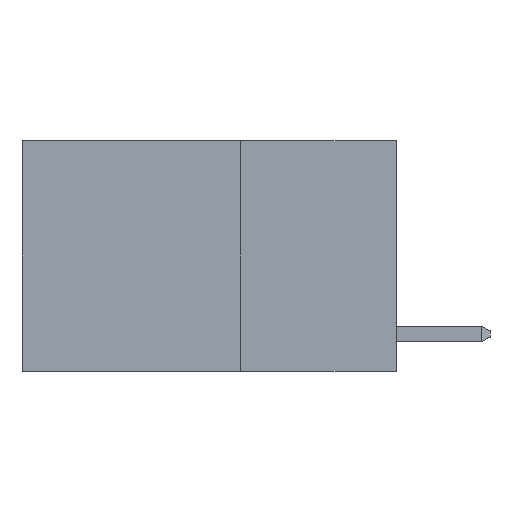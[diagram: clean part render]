
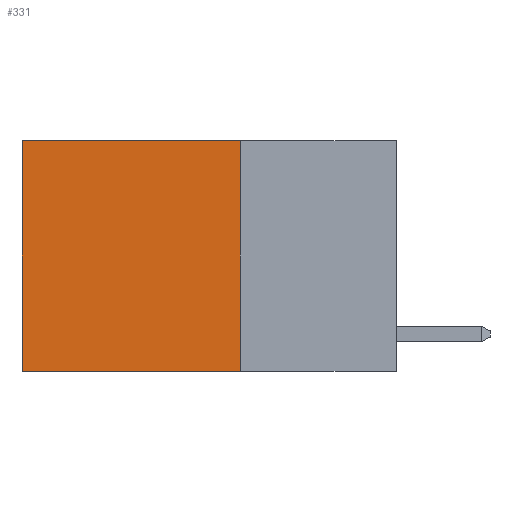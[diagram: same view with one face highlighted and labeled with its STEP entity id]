
A CAD part, left-side view. The second image highlights one B-rep face of the part: STEP entity #331.
In plain terms, the highlighted planar face has unit normal (-1, 0, 0).
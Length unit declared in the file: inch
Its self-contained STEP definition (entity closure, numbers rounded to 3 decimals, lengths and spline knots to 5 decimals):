
#331 = ADVANCED_FACE ( 'NONE', ( #4762 ), #3990, .F. ) ;
#354 = DIRECTION ( 'NONE',  ( 0., 0., -1. ) ) ;
#567 = CARTESIAN_POINT ( 'NONE',  ( 0.2625, 0.25, 0. ) ) ;
#941 = VERTEX_POINT ( 'NONE', #567 ) ;
#1017 = LINE ( 'NONE', #2188, #1271 ) ;
#1229 = EDGE_LOOP ( 'NONE', ( #3267, #4927, #3034, #3205 ) ) ;
#1271 = VECTOR ( 'NONE', #3035, 39.37008 ) ;
#1307 = VERTEX_POINT ( 'NONE', #6038 ) ;
#2188 = CARTESIAN_POINT ( 'NONE',  ( 0.2625, 0.25, 0. ) ) ;
#3005 = VECTOR ( 'NONE', #6098, 39.37008 ) ;
#3034 = ORIENTED_EDGE ( 'NONE', *, *, #4002, .F. ) ;
#3035 = DIRECTION ( 'NONE',  ( 0., 1., 0. ) ) ;
#3205 = ORIENTED_EDGE ( 'NONE', *, *, #7578, .T. ) ;
#3267 = ORIENTED_EDGE ( 'NONE', *, *, #6800, .T. ) ;
#3848 = DIRECTION ( 'NONE',  ( 0., 0., -1. ) ) ;
#3990 = PLANE ( 'NONE',  #9559 ) ;
#4002 = EDGE_CURVE ( 'NONE', #941, #1307, #10956, .T. ) ;
#4071 = CARTESIAN_POINT ( 'NONE',  ( 0.2625, 0.25, 0. ) ) ;
#4214 = CARTESIAN_POINT ( 'NONE',  ( 0.2625, 0.25, 0. ) ) ;
#4451 = VECTOR ( 'NONE', #354, 39.37008 ) ;
#4762 = FACE_OUTER_BOUND ( 'NONE', #1229, .T. ) ;
#4889 = DIRECTION ( 'NONE',  ( 1., 0., 0. ) ) ;
#4927 = ORIENTED_EDGE ( 'NONE', *, *, #9029, .F. ) ;
#6038 = CARTESIAN_POINT ( 'NONE',  ( 0.2625, 0.25, -0.37 ) ) ;
#6098 = DIRECTION ( 'NONE',  ( 0., 1., 0. ) ) ;
#6320 = CARTESIAN_POINT ( 'NONE',  ( 0.2625, 0.6, -0.37 ) ) ;
#6677 = LINE ( 'NONE', #10550, #4451 ) ;
#6772 = CARTESIAN_POINT ( 'NONE',  ( 0.2625, 0.6, 0. ) ) ;
#6800 = EDGE_CURVE ( 'NONE', #7800, #8593, #6677, .T. ) ;
#6942 = CARTESIAN_POINT ( 'NONE',  ( 0.2625, 0.25, -0.37 ) ) ;
#7578 = EDGE_CURVE ( 'NONE', #941, #7800, #1017, .T. ) ;
#7800 = VERTEX_POINT ( 'NONE', #6772 ) ;
#8593 = VERTEX_POINT ( 'NONE', #6320 ) ;
#8612 = VECTOR ( 'NONE', #10963, 39.37008 ) ;
#9029 = EDGE_CURVE ( 'NONE', #1307, #8593, #9792, .T. ) ;
#9559 = AXIS2_PLACEMENT_3D ( 'NONE', #4214, #4889, #3848 ) ;
#9792 = LINE ( 'NONE', #6942, #3005 ) ;
#10550 = CARTESIAN_POINT ( 'NONE',  ( 0.2625, 0.6, 0. ) ) ;
#10956 = LINE ( 'NONE', #4071, #8612 ) ;
#10963 = DIRECTION ( 'NONE',  ( 0., 0., -1. ) ) ;
